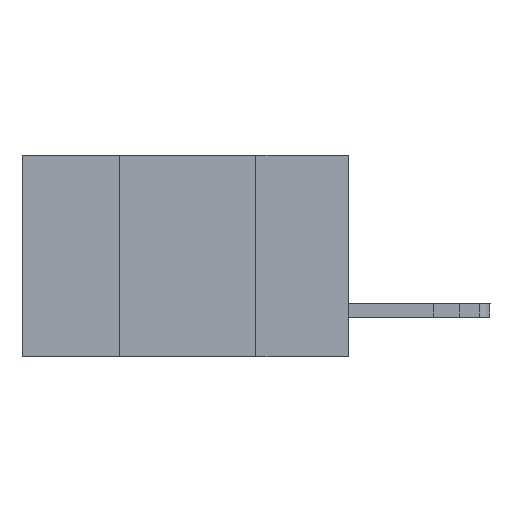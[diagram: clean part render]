
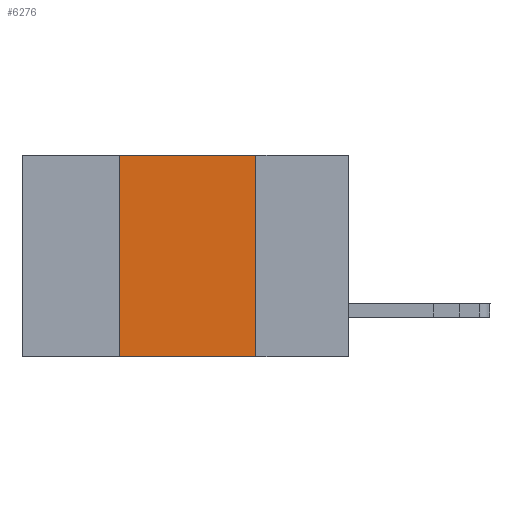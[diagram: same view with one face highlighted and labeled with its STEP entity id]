
A CAD part, left-side view. The second image highlights one B-rep face of the part: STEP entity #6276.
In plain terms, the highlighted planar face has unit normal (-1, 0, 0).
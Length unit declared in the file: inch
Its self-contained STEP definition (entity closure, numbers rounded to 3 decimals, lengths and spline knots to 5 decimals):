
#88 = CARTESIAN_POINT ( 'NONE',  ( 0., 0.6, -0.37 ) ) ;
#458 = CARTESIAN_POINT ( 'NONE',  ( 0., 0.6, 0. ) ) ;
#1276 = EDGE_LOOP ( 'NONE', ( #11801, #14656, #8571, #13948 ) ) ;
#1686 = DIRECTION ( 'NONE',  ( 0., 0., 1. ) ) ;
#1700 = PLANE ( 'NONE',  #8730 ) ;
#1737 = CARTESIAN_POINT ( 'NONE',  ( 0., 0.42, -0.37 ) ) ;
#2638 = EDGE_CURVE ( 'NONE', #11184, #13544, #6469, .T. ) ;
#2796 = CARTESIAN_POINT ( 'NONE',  ( 0., 0.42, 0. ) ) ;
#2818 = VERTEX_POINT ( 'NONE', #14718 ) ;
#3002 = LINE ( 'NONE', #9462, #13320 ) ;
#3829 = VECTOR ( 'NONE', #11509, 39.37008 ) ;
#4699 = CARTESIAN_POINT ( 'NONE',  ( 0., 0.17, -0.37 ) ) ;
#6168 = CARTESIAN_POINT ( 'NONE',  ( 0., 0.17, 0. ) ) ;
#6276 = ADVANCED_FACE ( 'NONE', ( #11793 ), #1700, .F. ) ;
#6469 = LINE ( 'NONE', #10514, #14102 ) ;
#7966 = EDGE_CURVE ( 'NONE', #9282, #11184, #3002, .T. ) ;
#8200 = EDGE_CURVE ( 'NONE', #9282, #2818, #11427, .T. ) ;
#8571 = ORIENTED_EDGE ( 'NONE', *, *, #7966, .F. ) ;
#8730 = AXIS2_PLACEMENT_3D ( 'NONE', #458, #12035, #9397 ) ;
#9282 = VERTEX_POINT ( 'NONE', #1737 ) ;
#9397 = DIRECTION ( 'NONE',  ( 0., 0., -1. ) ) ;
#9462 = CARTESIAN_POINT ( 'NONE',  ( 0., 0.42, -0.37 ) ) ;
#9989 = EDGE_CURVE ( 'NONE', #13544, #2818, #11054, .T. ) ;
#10514 = CARTESIAN_POINT ( 'NONE',  ( 0., 0.6, 0. ) ) ;
#10813 = DIRECTION ( 'NONE',  ( 0., 0., -1. ) ) ;
#11054 = LINE ( 'NONE', #4699, #12850 ) ;
#11184 = VERTEX_POINT ( 'NONE', #2796 ) ;
#11427 = LINE ( 'NONE', #88, #3829 ) ;
#11509 = DIRECTION ( 'NONE',  ( 0., -1., 0. ) ) ;
#11793 = FACE_OUTER_BOUND ( 'NONE', #1276, .T. ) ;
#11801 = ORIENTED_EDGE ( 'NONE', *, *, #9989, .F. ) ;
#12035 = DIRECTION ( 'NONE',  ( 1., 0., 0. ) ) ;
#12850 = VECTOR ( 'NONE', #10813, 39.37008 ) ;
#13320 = VECTOR ( 'NONE', #1686, 39.37008 ) ;
#13544 = VERTEX_POINT ( 'NONE', #6168 ) ;
#13948 = ORIENTED_EDGE ( 'NONE', *, *, #8200, .T. ) ;
#14102 = VECTOR ( 'NONE', #15535, 39.37008 ) ;
#14656 = ORIENTED_EDGE ( 'NONE', *, *, #2638, .F. ) ;
#14718 = CARTESIAN_POINT ( 'NONE',  ( 0., 0.17, -0.37 ) ) ;
#15535 = DIRECTION ( 'NONE',  ( 0., -1., 0. ) ) ;
